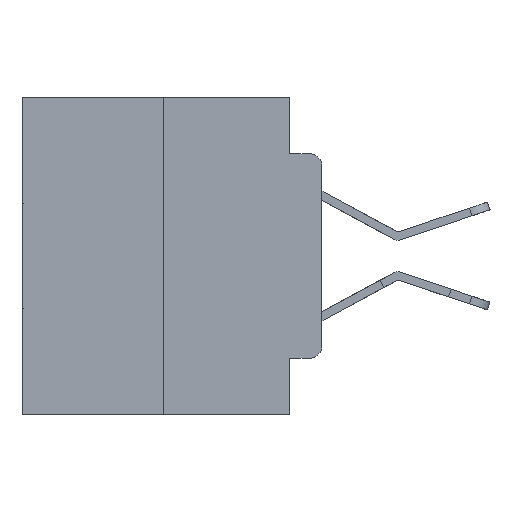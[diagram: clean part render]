
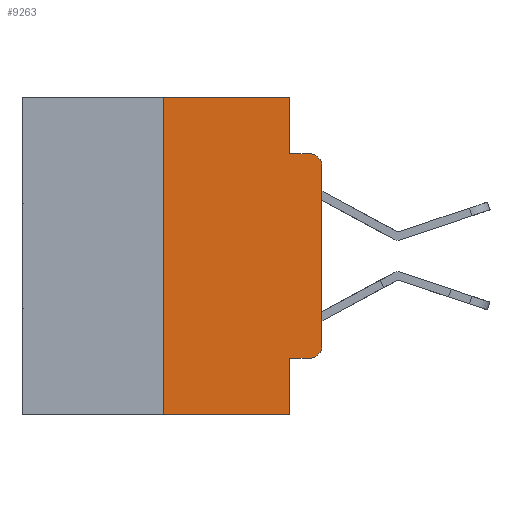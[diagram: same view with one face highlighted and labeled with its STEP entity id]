
A CAD part, left-side view. The second image highlights one B-rep face of the part: STEP entity #9263.
In plain terms, the highlighted planar face has unit normal (-1, 0, 0).
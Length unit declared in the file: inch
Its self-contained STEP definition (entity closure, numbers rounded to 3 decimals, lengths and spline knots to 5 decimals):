
#185 = ORIENTED_EDGE ( 'NONE', *, *, #20720, .F. ) ;
#286 = DIRECTION ( 'NONE',  ( -1., 0., 0. ) ) ;
#325 = DIRECTION ( 'NONE',  ( 1., 0., 0. ) ) ;
#368 = CARTESIAN_POINT ( 'NONE',  ( 0., 0., 0. ) ) ;
#1261 = PLANE ( 'NONE',  #21264 ) ;
#1924 = CARTESIAN_POINT ( 'NONE',  ( 0., 0.25, -0.5 ) ) ;
#2149 = LINE ( 'NONE', #368, #26796 ) ;
#2697 = AXIS2_PLACEMENT_3D ( 'NONE', #20274, #9692, #3086 ) ;
#2809 = VECTOR ( 'NONE', #26145, 39.37008 ) ;
#2949 = LINE ( 'NONE', #15806, #20530 ) ;
#2971 = CIRCLE ( 'NONE', #2697, 0.02 ) ;
#3086 = DIRECTION ( 'NONE',  ( 0., 0., -1. ) ) ;
#4079 = LINE ( 'NONE', #6910, #13882 ) ;
#4499 = VERTEX_POINT ( 'NONE', #1924 ) ;
#4696 = DIRECTION ( 'NONE',  ( 0., 0., -1. ) ) ;
#4910 = ORIENTED_EDGE ( 'NONE', *, *, #20768, .T. ) ;
#4980 = DIRECTION ( 'NONE',  ( 0., 0., -1. ) ) ;
#6312 = LINE ( 'NONE', #10807, #25876 ) ;
#6910 = CARTESIAN_POINT ( 'NONE',  ( 0., 0.051, 0. ) ) ;
#7928 = EDGE_CURVE ( 'NONE', #9623, #24100, #4079, .T. ) ;
#7945 = ORIENTED_EDGE ( 'NONE', *, *, #19784, .T. ) ;
#8955 = VERTEX_POINT ( 'NONE', #21108 ) ;
#9263 = ADVANCED_FACE ( 'NONE', ( #19185 ), #1261, .F. ) ;
#9623 = VERTEX_POINT ( 'NONE', #9871 ) ;
#9692 = DIRECTION ( 'NONE',  ( -1., 0., 0. ) ) ;
#9871 = CARTESIAN_POINT ( 'NONE',  ( 0., 0.051, 0. ) ) ;
#10807 = CARTESIAN_POINT ( 'NONE',  ( 0., 0.051, -0.0885 ) ) ;
#11243 = EDGE_CURVE ( 'NONE', #12210, #8955, #2149, .T. ) ;
#11370 = VERTEX_POINT ( 'NONE', #22618 ) ;
#11526 = CARTESIAN_POINT ( 'NONE',  ( 0., 0.02, -0.1085 ) ) ;
#11562 = VECTOR ( 'NONE', #11735, 39.37008 ) ;
#11735 = DIRECTION ( 'NONE',  ( 0., 0., 1. ) ) ;
#12098 = VERTEX_POINT ( 'NONE', #23544 ) ;
#12210 = VERTEX_POINT ( 'NONE', #23029 ) ;
#13047 = ORIENTED_EDGE ( 'NONE', *, *, #11243, .T. ) ;
#13882 = VECTOR ( 'NONE', #22214, 39.37008 ) ;
#14085 = DIRECTION ( 'NONE',  ( 0., -1., 0. ) ) ;
#14707 = ORIENTED_EDGE ( 'NONE', *, *, #25965, .F. ) ;
#14933 = ORIENTED_EDGE ( 'NONE', *, *, #27392, .F. ) ;
#14983 = LINE ( 'NONE', #21750, #2809 ) ;
#15678 = CARTESIAN_POINT ( 'NONE',  ( 0., 0.051, -0.4115 ) ) ;
#15806 = CARTESIAN_POINT ( 'NONE',  ( 0., 0.473, 0. ) ) ;
#15914 = VECTOR ( 'NONE', #14085, 39.37008 ) ;
#16838 = VERTEX_POINT ( 'NONE', #17014 ) ;
#17014 = CARTESIAN_POINT ( 'NONE',  ( 0., 0.25, 0. ) ) ;
#17248 = LINE ( 'NONE', #18415, #11562 ) ;
#17294 = DIRECTION ( 'NONE',  ( 0., -1., 0. ) ) ;
#18129 = CARTESIAN_POINT ( 'NONE',  ( 0., 0.473, -0.5 ) ) ;
#18415 = CARTESIAN_POINT ( 'NONE',  ( 0., 0.25, 0. ) ) ;
#18826 = VERTEX_POINT ( 'NONE', #25183 ) ;
#18880 = CARTESIAN_POINT ( 'NONE',  ( 0., 0.051, -0.0885 ) ) ;
#19183 = VECTOR ( 'NONE', #19258, 39.37008 ) ;
#19185 = FACE_OUTER_BOUND ( 'NONE', #22480, .T. ) ;
#19258 = DIRECTION ( 'NONE',  ( 0., 0., -1. ) ) ;
#19309 = CARTESIAN_POINT ( 'NONE',  ( 0., 0.473, 0. ) ) ;
#19784 = EDGE_CURVE ( 'NONE', #26651, #18826, #14983, .T. ) ;
#19928 = ORIENTED_EDGE ( 'NONE', *, *, #7928, .F. ) ;
#20083 = ORIENTED_EDGE ( 'NONE', *, *, #27191, .F. ) ;
#20274 = CARTESIAN_POINT ( 'NONE',  ( 0., 0.02, -0.3915 ) ) ;
#20530 = VECTOR ( 'NONE', #24299, 39.37008 ) ;
#20720 = EDGE_CURVE ( 'NONE', #4499, #16838, #17248, .T. ) ;
#20768 = EDGE_CURVE ( 'NONE', #4499, #12098, #21657, .T. ) ;
#20778 = ORIENTED_EDGE ( 'NONE', *, *, #26781, .T. ) ;
#21108 = CARTESIAN_POINT ( 'NONE',  ( 0., 0., -0.1085 ) ) ;
#21264 = AXIS2_PLACEMENT_3D ( 'NONE', #19309, #325, #4980 ) ;
#21657 = LINE ( 'NONE', #18129, #15914 ) ;
#21750 = CARTESIAN_POINT ( 'NONE',  ( 0., 0.051, -0.4115 ) ) ;
#22214 = DIRECTION ( 'NONE',  ( 0., 0., -1. ) ) ;
#22480 = EDGE_LOOP ( 'NONE', ( #13047, #27028, #20083, #19928, #14933, #185, #4910, #14707, #7945, #20778 ) ) ;
#22581 = LINE ( 'NONE', #27917, #19183 ) ;
#22618 = CARTESIAN_POINT ( 'NONE',  ( 0., 0.02, -0.0885 ) ) ;
#22990 = EDGE_CURVE ( 'NONE', #8955, #11370, #23568, .T. ) ;
#23029 = CARTESIAN_POINT ( 'NONE',  ( 0., 0., -0.3915 ) ) ;
#23544 = CARTESIAN_POINT ( 'NONE',  ( 0., 0.051, -0.5 ) ) ;
#23568 = CIRCLE ( 'NONE', #25935, 0.02 ) ;
#24100 = VERTEX_POINT ( 'NONE', #18880 ) ;
#24299 = DIRECTION ( 'NONE',  ( 0., -1., 0. ) ) ;
#25183 = CARTESIAN_POINT ( 'NONE',  ( 0., 0.02, -0.4115 ) ) ;
#25876 = VECTOR ( 'NONE', #17294, 39.37008 ) ;
#25935 = AXIS2_PLACEMENT_3D ( 'NONE', #11526, #286, #4696 ) ;
#25965 = EDGE_CURVE ( 'NONE', #26651, #12098, #22581, .T. ) ;
#26145 = DIRECTION ( 'NONE',  ( 0., -1., 0. ) ) ;
#26574 = DIRECTION ( 'NONE',  ( 0., 0., 1. ) ) ;
#26651 = VERTEX_POINT ( 'NONE', #15678 ) ;
#26781 = EDGE_CURVE ( 'NONE', #18826, #12210, #2971, .T. ) ;
#26796 = VECTOR ( 'NONE', #26574, 39.37008 ) ;
#27028 = ORIENTED_EDGE ( 'NONE', *, *, #22990, .T. ) ;
#27191 = EDGE_CURVE ( 'NONE', #24100, #11370, #6312, .T. ) ;
#27392 = EDGE_CURVE ( 'NONE', #16838, #9623, #2949, .T. ) ;
#27917 = CARTESIAN_POINT ( 'NONE',  ( 0., 0.051, 0. ) ) ;
